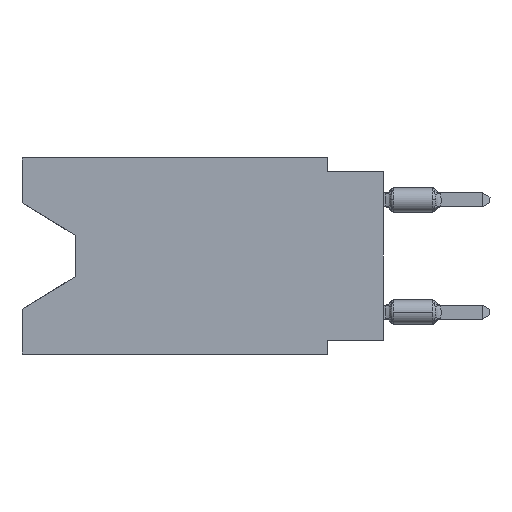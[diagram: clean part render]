
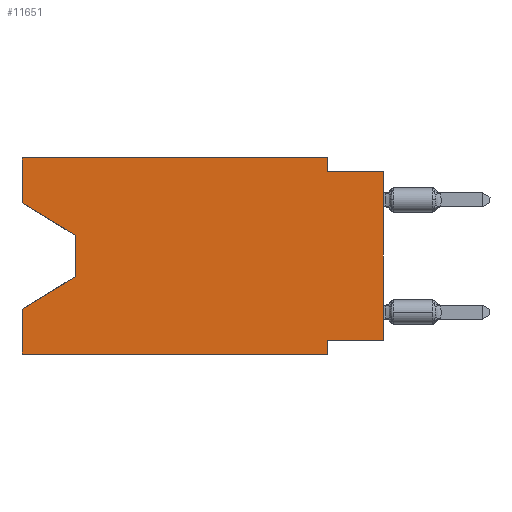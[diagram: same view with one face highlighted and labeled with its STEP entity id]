
A CAD part, left-side view. The second image highlights one B-rep face of the part: STEP entity #11651.
In plain terms, the highlighted planar face has unit normal (-1, 0, 0).
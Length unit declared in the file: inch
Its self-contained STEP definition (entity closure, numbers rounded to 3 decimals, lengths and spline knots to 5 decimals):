
#115 = LINE ( 'NONE', #7074, #6693 ) ;
#658 = CARTESIAN_POINT ( 'NONE',  ( 0., 0.1, 0. ) ) ;
#880 = CARTESIAN_POINT ( 'NONE',  ( 0., 0., -0.025 ) ) ;
#1008 = VERTEX_POINT ( 'NONE', #6086 ) ;
#1470 = CARTESIAN_POINT ( 'NONE',  ( 0., 0.1, -0.35 ) ) ;
#1523 = EDGE_CURVE ( 'NONE', #7226, #7380, #7055, .T. ) ;
#1696 = ORIENTED_EDGE ( 'NONE', *, *, #1523, .T. ) ;
#2019 = CARTESIAN_POINT ( 'NONE',  ( 0., 0.55, -0.138 ) ) ;
#2087 = CARTESIAN_POINT ( 'NONE',  ( 0., 0.55, -0.212 ) ) ;
#2268 = LINE ( 'NONE', #7146, #4969 ) ;
#2279 = ORIENTED_EDGE ( 'NONE', *, *, #15888, .T. ) ;
#2506 = ORIENTED_EDGE ( 'NONE', *, *, #3411, .F. ) ;
#2522 = CARTESIAN_POINT ( 'NONE',  ( 0., 0.645, 0. ) ) ;
#2596 = CARTESIAN_POINT ( 'NONE',  ( 0., 0.1, -0.025 ) ) ;
#3150 = ORIENTED_EDGE ( 'NONE', *, *, #13177, .F. ) ;
#3198 = AXIS2_PLACEMENT_3D ( 'NONE', #7589, #11503, #8706 ) ;
#3218 = VECTOR ( 'NONE', #14699, 39.37008 ) ;
#3258 = VERTEX_POINT ( 'NONE', #11954 ) ;
#3411 = EDGE_CURVE ( 'NONE', #1008, #4696, #5390, .T. ) ;
#3563 = EDGE_CURVE ( 'NONE', #11796, #7226, #11587, .T. ) ;
#3571 = VECTOR ( 'NONE', #11849, 39.37008 ) ;
#3803 = EDGE_CURVE ( 'NONE', #5577, #3258, #14303, .T. ) ;
#3830 = FACE_OUTER_BOUND ( 'NONE', #15027, .T. ) ;
#3915 = CARTESIAN_POINT ( 'NONE',  ( 0., 0.645, -0.08025 ) ) ;
#4071 = ORIENTED_EDGE ( 'NONE', *, *, #6996, .F. ) ;
#4429 = VECTOR ( 'NONE', #12950, 39.37008 ) ;
#4527 = CARTESIAN_POINT ( 'NONE',  ( 0., 0., 0. ) ) ;
#4696 = VERTEX_POINT ( 'NONE', #16301 ) ;
#4778 = ORIENTED_EDGE ( 'NONE', *, *, #9855, .F. ) ;
#4917 = CARTESIAN_POINT ( 'NONE',  ( 0., 0., -0.325 ) ) ;
#4969 = VECTOR ( 'NONE', #13684, 39.37008 ) ;
#5262 = ORIENTED_EDGE ( 'NONE', *, *, #15759, .T. ) ;
#5283 = DIRECTION ( 'NONE',  ( 0., 1., 0. ) ) ;
#5390 = LINE ( 'NONE', #10594, #13400 ) ;
#5577 = VERTEX_POINT ( 'NONE', #15822 ) ;
#5833 = DIRECTION ( 'NONE',  ( 0., 0., -1. ) ) ;
#6002 = DIRECTION ( 'NONE',  ( 0., 0.855, -0.519 ) ) ;
#6086 = CARTESIAN_POINT ( 'NONE',  ( 0., 0.645, -0.35 ) ) ;
#6432 = VECTOR ( 'NONE', #9690, 39.37008 ) ;
#6693 = VECTOR ( 'NONE', #5283, 39.37008 ) ;
#6784 = EDGE_CURVE ( 'NONE', #14443, #5577, #115, .T. ) ;
#6996 = EDGE_CURVE ( 'NONE', #11796, #15783, #11470, .T. ) ;
#7055 = LINE ( 'NONE', #2019, #6432 ) ;
#7074 = CARTESIAN_POINT ( 'NONE',  ( 0., 0., -0.325 ) ) ;
#7146 = CARTESIAN_POINT ( 'NONE',  ( 0., 0.645, 0. ) ) ;
#7226 = VERTEX_POINT ( 'NONE', #8484 ) ;
#7308 = VECTOR ( 'NONE', #6002, 39.37008 ) ;
#7380 = VERTEX_POINT ( 'NONE', #11944 ) ;
#7589 = CARTESIAN_POINT ( 'NONE',  ( 0., 0.645, 0. ) ) ;
#8126 = VERTEX_POINT ( 'NONE', #2596 ) ;
#8251 = VECTOR ( 'NONE', #13384, 39.37008 ) ;
#8484 = CARTESIAN_POINT ( 'NONE',  ( 0., 0.55, -0.138 ) ) ;
#8706 = DIRECTION ( 'NONE',  ( 0., 0., -1. ) ) ;
#8920 = DIRECTION ( 'NONE',  ( 0., 0., 1. ) ) ;
#9046 = CARTESIAN_POINT ( 'NONE',  ( 0., 0.645, -0.08025 ) ) ;
#9334 = ORIENTED_EDGE ( 'NONE', *, *, #15359, .F. ) ;
#9690 = DIRECTION ( 'NONE',  ( 0., 0., -1. ) ) ;
#9756 = CARTESIAN_POINT ( 'NONE',  ( 0., 0.1, 0. ) ) ;
#9855 = EDGE_CURVE ( 'NONE', #12416, #8126, #13654, .T. ) ;
#10594 = CARTESIAN_POINT ( 'NONE',  ( 0., 0.645, 0. ) ) ;
#10779 = LINE ( 'NONE', #15964, #3218 ) ;
#11016 = ORIENTED_EDGE ( 'NONE', *, *, #3563, .T. ) ;
#11117 = CARTESIAN_POINT ( 'NONE',  ( 0., 0.645, 0. ) ) ;
#11470 = LINE ( 'NONE', #2522, #11577 ) ;
#11503 = DIRECTION ( 'NONE',  ( 1., 0., 0. ) ) ;
#11577 = VECTOR ( 'NONE', #8920, 39.37008 ) ;
#11587 = LINE ( 'NONE', #9046, #4429 ) ;
#11651 = ADVANCED_FACE ( 'NONE', ( #3830 ), #16607, .F. ) ;
#11796 = VERTEX_POINT ( 'NONE', #3915 ) ;
#11849 = DIRECTION ( 'NONE',  ( 0., 0., -1. ) ) ;
#11944 = CARTESIAN_POINT ( 'NONE',  ( 0., 0.55, -0.212 ) ) ;
#11954 = CARTESIAN_POINT ( 'NONE',  ( 0., 0.1, -0.35 ) ) ;
#12416 = VERTEX_POINT ( 'NONE', #9756 ) ;
#12950 = DIRECTION ( 'NONE',  ( 0., -0.855, -0.519 ) ) ;
#13177 = EDGE_CURVE ( 'NONE', #8126, #14063, #14569, .T. ) ;
#13384 = DIRECTION ( 'NONE',  ( 0., 0., 1. ) ) ;
#13400 = VECTOR ( 'NONE', #15785, 39.37008 ) ;
#13654 = LINE ( 'NONE', #658, #16527 ) ;
#13675 = VECTOR ( 'NONE', #16013, 39.37008 ) ;
#13684 = DIRECTION ( 'NONE',  ( 0., -1., 0. ) ) ;
#13749 = LINE ( 'NONE', #2087, #7308 ) ;
#13807 = ORIENTED_EDGE ( 'NONE', *, *, #15004, .T. ) ;
#14063 = VERTEX_POINT ( 'NONE', #880 ) ;
#14303 = LINE ( 'NONE', #1470, #3571 ) ;
#14443 = VERTEX_POINT ( 'NONE', #4917 ) ;
#14569 = LINE ( 'NONE', #14655, #13675 ) ;
#14655 = CARTESIAN_POINT ( 'NONE',  ( 0., 0., -0.025 ) ) ;
#14699 = DIRECTION ( 'NONE',  ( 0., -1., 0. ) ) ;
#14712 = ORIENTED_EDGE ( 'NONE', *, *, #3803, .F. ) ;
#14894 = ORIENTED_EDGE ( 'NONE', *, *, #6784, .F. ) ;
#15004 = EDGE_CURVE ( 'NONE', #14443, #14063, #16029, .T. ) ;
#15027 = EDGE_LOOP ( 'NONE', ( #11016, #1696, #2279, #2506, #5262, #14712, #14894, #13807, #3150, #4778, #9334, #4071 ) ) ;
#15359 = EDGE_CURVE ( 'NONE', #15783, #12416, #2268, .T. ) ;
#15759 = EDGE_CURVE ( 'NONE', #1008, #3258, #10779, .T. ) ;
#15783 = VERTEX_POINT ( 'NONE', #11117 ) ;
#15785 = DIRECTION ( 'NONE',  ( 0., 0., 1. ) ) ;
#15822 = CARTESIAN_POINT ( 'NONE',  ( 0., 0.1, -0.325 ) ) ;
#15888 = EDGE_CURVE ( 'NONE', #7380, #4696, #13749, .T. ) ;
#15964 = CARTESIAN_POINT ( 'NONE',  ( 0., 0.645, -0.35 ) ) ;
#16013 = DIRECTION ( 'NONE',  ( 0., -1., 0. ) ) ;
#16029 = LINE ( 'NONE', #4527, #8251 ) ;
#16301 = CARTESIAN_POINT ( 'NONE',  ( 0., 0.645, -0.26975 ) ) ;
#16527 = VECTOR ( 'NONE', #5833, 39.37008 ) ;
#16607 = PLANE ( 'NONE',  #3198 ) ;
